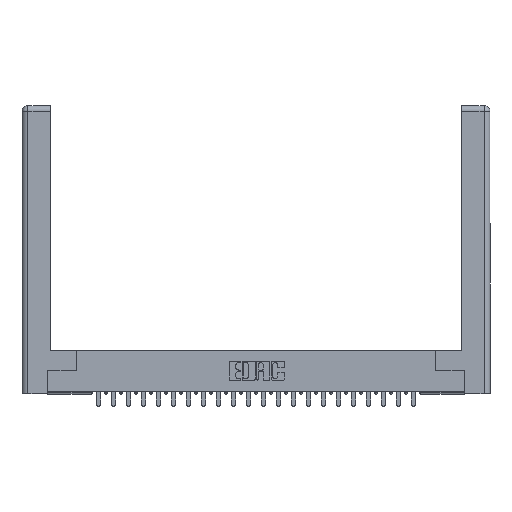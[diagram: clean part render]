
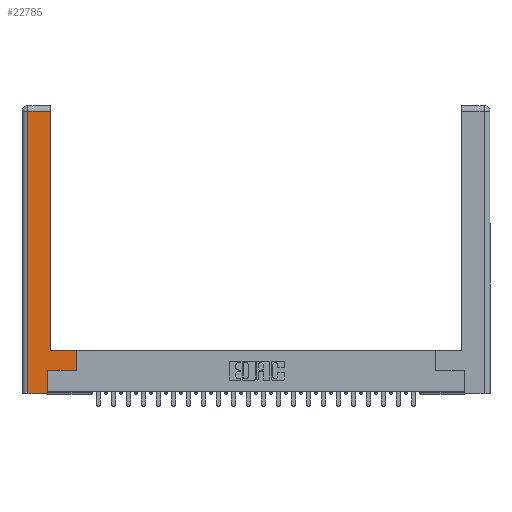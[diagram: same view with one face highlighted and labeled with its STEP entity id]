
A CAD part, top view. The second image highlights one B-rep face of the part: STEP entity #22785.
In plain terms, the highlighted planar face has unit normal (0, 0, 1).
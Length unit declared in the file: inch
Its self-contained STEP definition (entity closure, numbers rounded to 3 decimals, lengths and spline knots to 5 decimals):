
#343 = VERTEX_POINT ( 'NONE', #10213 ) ;
#465 = EDGE_CURVE ( 'NONE', #28149, #16379, #21047, .T. ) ;
#968 = DIRECTION ( 'NONE',  ( 0., 1., 0. ) ) ;
#3313 = VECTOR ( 'NONE', #968, 39.37008 ) ;
#4391 = CARTESIAN_POINT ( 'NONE',  ( 0.265, 0.245, 0. ) ) ;
#4818 = DIRECTION ( 'NONE',  ( 0., -1., 0. ) ) ;
#5759 = VECTOR ( 'NONE', #28660, 39.37008 ) ;
#6222 = LINE ( 'NONE', #21559, #27443 ) ;
#6305 = ORIENTED_EDGE ( 'NONE', *, *, #28038, .T. ) ;
#7049 = CARTESIAN_POINT ( 'NONE',  ( 0.295, 0.45, 0. ) ) ;
#9062 = EDGE_CURVE ( 'NONE', #16379, #10194, #25402, .T. ) ;
#9110 = CARTESIAN_POINT ( 'NONE',  ( 0.265, 0., 0. ) ) ;
#9122 = VERTEX_POINT ( 'NONE', #20556 ) ;
#9208 = CARTESIAN_POINT ( 'NONE',  ( 0.0615, 2.94, 0. ) ) ;
#9767 = VERTEX_POINT ( 'NONE', #9208 ) ;
#10011 = VERTEX_POINT ( 'NONE', #19832 ) ;
#10012 = EDGE_CURVE ( 'NONE', #17612, #28149, #13181, .T. ) ;
#10194 = VERTEX_POINT ( 'NONE', #23373 ) ;
#10213 = CARTESIAN_POINT ( 'NONE',  ( 0.265, 0., 0. ) ) ;
#11439 = ORIENTED_EDGE ( 'NONE', *, *, #465, .T. ) ;
#11516 = VECTOR ( 'NONE', #13562, 39.37008 ) ;
#11624 = CARTESIAN_POINT ( 'NONE',  ( 0.565, 0.245, 0. ) ) ;
#11970 = LINE ( 'NONE', #9110, #20342 ) ;
#12541 = ORIENTED_EDGE ( 'NONE', *, *, #10012, .T. ) ;
#13181 = LINE ( 'NONE', #27100, #21507 ) ;
#13562 = DIRECTION ( 'NONE',  ( -1., 0., 0. ) ) ;
#15151 = ORIENTED_EDGE ( 'NONE', *, *, #22377, .T. ) ;
#15298 = FACE_OUTER_BOUND ( 'NONE', #15764, .T. ) ;
#15658 = AXIS2_PLACEMENT_3D ( 'NONE', #16587, #21048, #16396 ) ;
#15764 = EDGE_LOOP ( 'NONE', ( #15151, #25860, #19303, #18724, #6305, #12541, #11439, #20517 ) ) ;
#16379 = VERTEX_POINT ( 'NONE', #17397 ) ;
#16396 = DIRECTION ( 'NONE',  ( -1., 0., 0. ) ) ;
#16512 = VECTOR ( 'NONE', #28350, 39.37008 ) ;
#16587 = CARTESIAN_POINT ( 'NONE',  ( 0., 0., 0. ) ) ;
#17284 = LINE ( 'NONE', #24282, #5759 ) ;
#17397 = CARTESIAN_POINT ( 'NONE',  ( 0.565, 0.45, 0. ) ) ;
#17571 = CARTESIAN_POINT ( 'NONE',  ( 0.0615, 2.94, 0. ) ) ;
#17612 = VERTEX_POINT ( 'NONE', #4391 ) ;
#18171 = VECTOR ( 'NONE', #4818, 39.37008 ) ;
#18724 = ORIENTED_EDGE ( 'NONE', *, *, #26260, .T. ) ;
#19303 = ORIENTED_EDGE ( 'NONE', *, *, #27411, .T. ) ;
#19832 = CARTESIAN_POINT ( 'NONE',  ( 0.0615, 0., 0. ) ) ;
#20056 = DIRECTION ( 'NONE',  ( 1., 0., 0. ) ) ;
#20342 = VECTOR ( 'NONE', #20056, 39.37008 ) ;
#20517 = ORIENTED_EDGE ( 'NONE', *, *, #9062, .T. ) ;
#20556 = CARTESIAN_POINT ( 'NONE',  ( 0.295, 2.94, 0. ) ) ;
#21047 = LINE ( 'NONE', #25230, #3313 ) ;
#21048 = DIRECTION ( 'NONE',  ( 0., 0., -1. ) ) ;
#21507 = VECTOR ( 'NONE', #22645, 39.37008 ) ;
#21559 = CARTESIAN_POINT ( 'NONE',  ( 0.295, 3., 0. ) ) ;
#21656 = DIRECTION ( 'NONE',  ( 0., 1., 0. ) ) ;
#22377 = EDGE_CURVE ( 'NONE', #10194, #9122, #6222, .T. ) ;
#22645 = DIRECTION ( 'NONE',  ( 1., 0., 0. ) ) ;
#22682 = LINE ( 'NONE', #24939, #18171 ) ;
#22785 = ADVANCED_FACE ( 'NONE', ( #15298 ), #25136, .F. ) ;
#23373 = CARTESIAN_POINT ( 'NONE',  ( 0.295, 0.45, 0. ) ) ;
#24282 = CARTESIAN_POINT ( 'NONE',  ( 0.265, 0.245, 0. ) ) ;
#24939 = CARTESIAN_POINT ( 'NONE',  ( 0.0615, 0., 0. ) ) ;
#25136 = PLANE ( 'NONE',  #15658 ) ;
#25210 = LINE ( 'NONE', #17571, #16512 ) ;
#25230 = CARTESIAN_POINT ( 'NONE',  ( 0.565, 0.45, 0. ) ) ;
#25402 = LINE ( 'NONE', #7049, #11516 ) ;
#25860 = ORIENTED_EDGE ( 'NONE', *, *, #25920, .T. ) ;
#25920 = EDGE_CURVE ( 'NONE', #9122, #9767, #25210, .T. ) ;
#26260 = EDGE_CURVE ( 'NONE', #10011, #343, #11970, .T. ) ;
#27100 = CARTESIAN_POINT ( 'NONE',  ( 0.565, 0.245, 0. ) ) ;
#27411 = EDGE_CURVE ( 'NONE', #9767, #10011, #22682, .T. ) ;
#27443 = VECTOR ( 'NONE', #21656, 39.37008 ) ;
#28038 = EDGE_CURVE ( 'NONE', #343, #17612, #17284, .T. ) ;
#28149 = VERTEX_POINT ( 'NONE', #11624 ) ;
#28350 = DIRECTION ( 'NONE',  ( -1., 0., 0. ) ) ;
#28660 = DIRECTION ( 'NONE',  ( 0., 1., 0. ) ) ;
